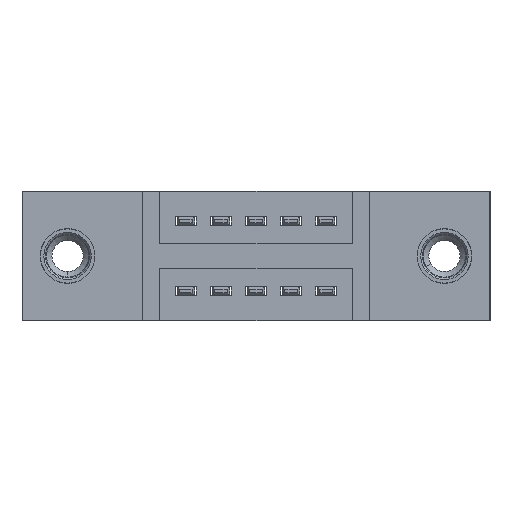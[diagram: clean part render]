
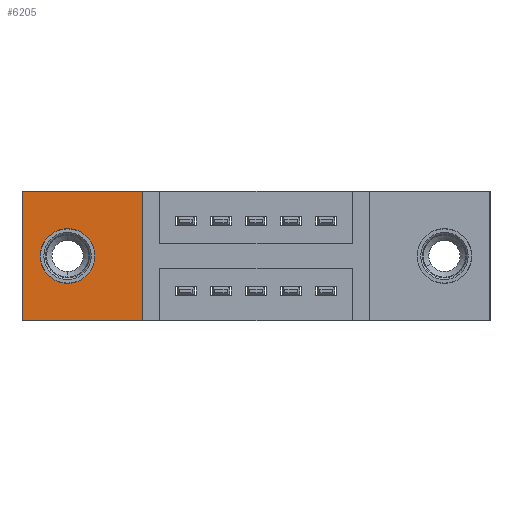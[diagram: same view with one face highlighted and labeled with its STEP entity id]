
A CAD part, front view. The second image highlights one B-rep face of the part: STEP entity #6205.
In plain terms, the highlighted planar face has unit normal (0, -1, 0).
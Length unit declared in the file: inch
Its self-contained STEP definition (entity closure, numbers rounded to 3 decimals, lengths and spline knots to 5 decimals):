
#382 = LINE ( 'NONE', #2704, #4143 ) ;
#409 = EDGE_CURVE ( 'NONE', #9546, #3671, #7613, .T. ) ;
#768 = CARTESIAN_POINT ( 'NONE',  ( 0.13, 0.17, -0.185 ) ) ;
#869 = CARTESIAN_POINT ( 'NONE',  ( 0., 0.17, -0.37 ) ) ;
#1090 = CARTESIAN_POINT ( 'NONE',  ( 0.13, 0.17, -0.263 ) ) ;
#1560 = DIRECTION ( 'NONE',  ( 0., -1., 0. ) ) ;
#1794 = CIRCLE ( 'NONE', #2442, 0.078 ) ;
#1917 = CARTESIAN_POINT ( 'NONE',  ( 0.3425, 0.17, -0.37 ) ) ;
#2373 = CARTESIAN_POINT ( 'NONE',  ( 0.3425, 0.17, 0. ) ) ;
#2416 = VECTOR ( 'NONE', #6308, 39.37008 ) ;
#2442 = AXIS2_PLACEMENT_3D ( 'NONE', #3966, #7063, #5626 ) ;
#2687 = AXIS2_PLACEMENT_3D ( 'NONE', #768, #1560, #8467 ) ;
#2704 = CARTESIAN_POINT ( 'NONE',  ( 0., 0.17, 0. ) ) ;
#2791 = CARTESIAN_POINT ( 'NONE',  ( 0., 0.17, 0. ) ) ;
#2812 = CARTESIAN_POINT ( 'NONE',  ( 0.13, 0.17, -0.107 ) ) ;
#2975 = EDGE_CURVE ( 'NONE', #7331, #9581, #382, .T. ) ;
#3355 = VECTOR ( 'NONE', #5468, 39.37008 ) ;
#3445 = EDGE_CURVE ( 'NONE', #8005, #4822, #7058, .T. ) ;
#3475 = LINE ( 'NONE', #2373, #3355 ) ;
#3478 = PLANE ( 'NONE',  #9425 ) ;
#3486 = LINE ( 'NONE', #2791, #7626 ) ;
#3671 = VERTEX_POINT ( 'NONE', #1917 ) ;
#3966 = CARTESIAN_POINT ( 'NONE',  ( 0.13, 0.17, -0.185 ) ) ;
#4143 = VECTOR ( 'NONE', #9661, 39.37008 ) ;
#4822 = VERTEX_POINT ( 'NONE', #2812 ) ;
#4929 = FACE_OUTER_BOUND ( 'NONE', #9663, .T. ) ;
#5111 = ORIENTED_EDGE ( 'NONE', *, *, #3445, .F. ) ;
#5263 = DIRECTION ( 'NONE',  ( 0., -1., 0. ) ) ;
#5407 = DIRECTION ( 'NONE',  ( 0., 0., -1. ) ) ;
#5468 = DIRECTION ( 'NONE',  ( 0., 0., 1. ) ) ;
#5626 = DIRECTION ( 'NONE',  ( 0., 0., -1. ) ) ;
#5935 = CARTESIAN_POINT ( 'NONE',  ( 0., 0.17, -0.37 ) ) ;
#6205 = ADVANCED_FACE ( 'NONE', ( #7130, #4929 ), #3478, .T. ) ;
#6308 = DIRECTION ( 'NONE',  ( 1., 0., 0. ) ) ;
#6338 = EDGE_CURVE ( 'NONE', #9581, #9546, #3486, .T. ) ;
#6426 = CARTESIAN_POINT ( 'NONE',  ( 0., 0.17, -0.37 ) ) ;
#6882 = EDGE_CURVE ( 'NONE', #4822, #8005, #1794, .T. ) ;
#6994 = EDGE_CURVE ( 'NONE', #3671, #7331, #3475, .T. ) ;
#7058 = CIRCLE ( 'NONE', #2687, 0.078 ) ;
#7063 = DIRECTION ( 'NONE',  ( 0., -1., 0. ) ) ;
#7130 = FACE_BOUND ( 'NONE', #9543, .T. ) ;
#7331 = VERTEX_POINT ( 'NONE', #9869 ) ;
#7527 = ORIENTED_EDGE ( 'NONE', *, *, #6994, .T. ) ;
#7568 = ORIENTED_EDGE ( 'NONE', *, *, #2975, .T. ) ;
#7613 = LINE ( 'NONE', #869, #2416 ) ;
#7626 = VECTOR ( 'NONE', #5407, 39.37008 ) ;
#8005 = VERTEX_POINT ( 'NONE', #1090 ) ;
#8200 = CARTESIAN_POINT ( 'NONE',  ( 0., 0.17, 0. ) ) ;
#8467 = DIRECTION ( 'NONE',  ( 0., 0., -1. ) ) ;
#9010 = ORIENTED_EDGE ( 'NONE', *, *, #6882, .F. ) ;
#9025 = ORIENTED_EDGE ( 'NONE', *, *, #6338, .T. ) ;
#9425 = AXIS2_PLACEMENT_3D ( 'NONE', #6426, #5263, #9755 ) ;
#9543 = EDGE_LOOP ( 'NONE', ( #9010, #5111 ) ) ;
#9546 = VERTEX_POINT ( 'NONE', #5935 ) ;
#9581 = VERTEX_POINT ( 'NONE', #8200 ) ;
#9593 = ORIENTED_EDGE ( 'NONE', *, *, #409, .T. ) ;
#9661 = DIRECTION ( 'NONE',  ( -1., 0., 0. ) ) ;
#9663 = EDGE_LOOP ( 'NONE', ( #9025, #9593, #7527, #7568 ) ) ;
#9755 = DIRECTION ( 'NONE',  ( 0., 0., -1. ) ) ;
#9869 = CARTESIAN_POINT ( 'NONE',  ( 0.3425, 0.17, 0. ) ) ;
